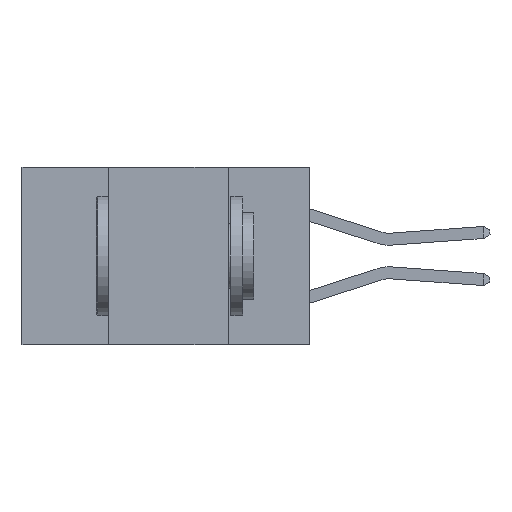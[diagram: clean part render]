
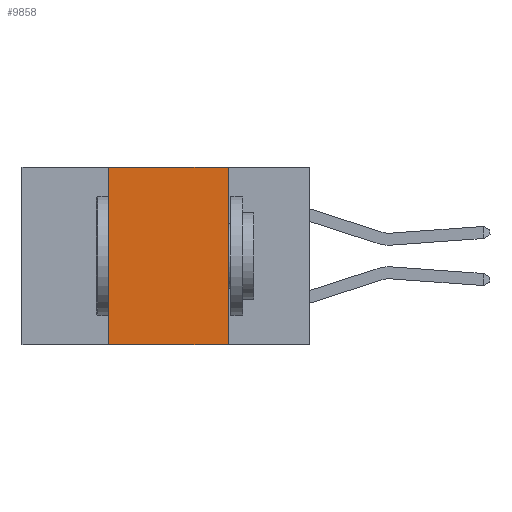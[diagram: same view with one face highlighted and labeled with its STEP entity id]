
A CAD part, left-side view. The second image highlights one B-rep face of the part: STEP entity #9858.
In plain terms, the highlighted planar face has unit normal (-1, 0, 0).
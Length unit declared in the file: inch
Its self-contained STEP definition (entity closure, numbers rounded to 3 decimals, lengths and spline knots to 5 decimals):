
#934 = VECTOR ( 'NONE', #8293, 39.37008 ) ;
#2027 = VERTEX_POINT ( 'NONE', #2359 ) ;
#2156 = CARTESIAN_POINT ( 'NONE',  ( 0., 0.6, 0. ) ) ;
#2201 = VERTEX_POINT ( 'NONE', #10342 ) ;
#2359 = CARTESIAN_POINT ( 'NONE',  ( 0., 0.42, -0.37 ) ) ;
#2825 = VECTOR ( 'NONE', #6279, 39.37008 ) ;
#2826 = CARTESIAN_POINT ( 'NONE',  ( 0., 0.6, 0. ) ) ;
#2959 = LINE ( 'NONE', #8218, #8478 ) ;
#3845 = DIRECTION ( 'NONE',  ( 0., -1., 0. ) ) ;
#3920 = LINE ( 'NONE', #12029, #934 ) ;
#3969 = DIRECTION ( 'NONE',  ( 0., -1., 0. ) ) ;
#5691 = EDGE_CURVE ( 'NONE', #8144, #2201, #3920, .T. ) ;
#6279 = DIRECTION ( 'NONE',  ( 0., 0., 1. ) ) ;
#6660 = PLANE ( 'NONE',  #12047 ) ;
#7755 = DIRECTION ( 'NONE',  ( 0., 0., -1. ) ) ;
#7949 = VERTEX_POINT ( 'NONE', #11492 ) ;
#7995 = EDGE_CURVE ( 'NONE', #2027, #7949, #11145, .T. ) ;
#8144 = VERTEX_POINT ( 'NONE', #13893 ) ;
#8218 = CARTESIAN_POINT ( 'NONE',  ( 0., 0.6, -0.37 ) ) ;
#8221 = LINE ( 'NONE', #2826, #13772 ) ;
#8293 = DIRECTION ( 'NONE',  ( 0., 0., -1. ) ) ;
#8478 = VECTOR ( 'NONE', #3845, 39.37008 ) ;
#8763 = ORIENTED_EDGE ( 'NONE', *, *, #9080, .T. ) ;
#9080 = EDGE_CURVE ( 'NONE', #2027, #2201, #2959, .T. ) ;
#9858 = ADVANCED_FACE ( 'NONE', ( #13348 ), #6660, .F. ) ;
#9885 = ORIENTED_EDGE ( 'NONE', *, *, #7995, .F. ) ;
#10342 = CARTESIAN_POINT ( 'NONE',  ( 0., 0.17, -0.37 ) ) ;
#10550 = ORIENTED_EDGE ( 'NONE', *, *, #10921, .F. ) ;
#10921 = EDGE_CURVE ( 'NONE', #7949, #8144, #8221, .T. ) ;
#11145 = LINE ( 'NONE', #12659, #2825 ) ;
#11492 = CARTESIAN_POINT ( 'NONE',  ( 0., 0.42, 0. ) ) ;
#12029 = CARTESIAN_POINT ( 'NONE',  ( 0., 0.17, 0. ) ) ;
#12047 = AXIS2_PLACEMENT_3D ( 'NONE', #2156, #14015, #7755 ) ;
#12659 = CARTESIAN_POINT ( 'NONE',  ( 0., 0.42, 0. ) ) ;
#12869 = ORIENTED_EDGE ( 'NONE', *, *, #5691, .F. ) ;
#13348 = FACE_OUTER_BOUND ( 'NONE', #13572, .T. ) ;
#13572 = EDGE_LOOP ( 'NONE', ( #12869, #10550, #9885, #8763 ) ) ;
#13772 = VECTOR ( 'NONE', #3969, 39.37008 ) ;
#13893 = CARTESIAN_POINT ( 'NONE',  ( 0., 0.17, 0. ) ) ;
#14015 = DIRECTION ( 'NONE',  ( 1., 0., 0. ) ) ;
